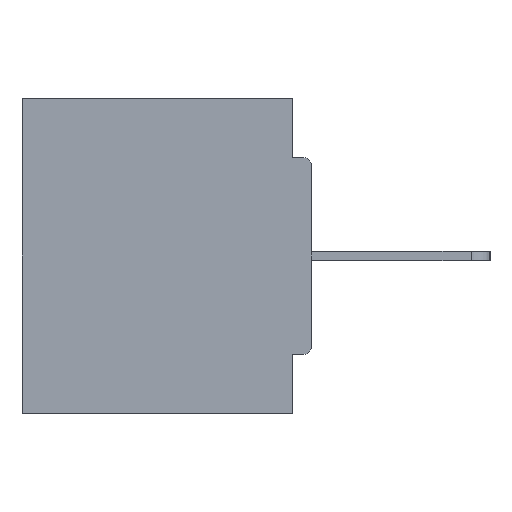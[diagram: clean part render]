
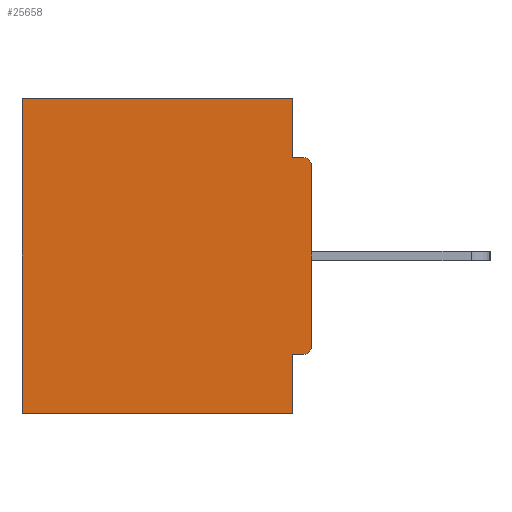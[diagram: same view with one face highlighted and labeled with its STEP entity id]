
A CAD part, left-side view. The second image highlights one B-rep face of the part: STEP entity #25658.
In plain terms, the highlighted planar face has unit normal (-1, 0, 0).
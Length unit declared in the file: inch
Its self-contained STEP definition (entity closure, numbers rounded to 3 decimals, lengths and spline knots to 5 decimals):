
#181 = ORIENTED_EDGE ( 'NONE', *, *, #11917, .T. ) ;
#790 = VECTOR ( 'NONE', #14850, 39.37008 ) ;
#1094 = VERTEX_POINT ( 'NONE', #14234 ) ;
#1147 = ORIENTED_EDGE ( 'NONE', *, *, #4278, .F. ) ;
#1227 = CARTESIAN_POINT ( 'NONE',  ( 0.298, 0., -0.0935 ) ) ;
#1301 = EDGE_CURVE ( 'NONE', #15742, #10105, #11719, .T. ) ;
#1604 = DIRECTION ( 'NONE',  ( -1., 0., 0. ) ) ;
#2246 = ORIENTED_EDGE ( 'NONE', *, *, #27350, .T. ) ;
#3933 = ORIENTED_EDGE ( 'NONE', *, *, #7257, .F. ) ;
#4278 = EDGE_CURVE ( 'NONE', #13126, #27658, #23858, .T. ) ;
#4291 = CARTESIAN_POINT ( 'NONE',  ( 0.298, 0.031, -0.5 ) ) ;
#4510 = DIRECTION ( 'NONE',  ( 0., 0., -1. ) ) ;
#5051 = CARTESIAN_POINT ( 'NONE',  ( 0.298, 0., 0. ) ) ;
#5140 = CIRCLE ( 'NONE', #22056, 0.015 ) ;
#5255 = DIRECTION ( 'NONE',  ( -1., 0., 0. ) ) ;
#5311 = CARTESIAN_POINT ( 'NONE',  ( 0.298, 0.015, -0.0935 ) ) ;
#5749 = EDGE_CURVE ( 'NONE', #11414, #7075, #10099, .T. ) ;
#6033 = FACE_OUTER_BOUND ( 'NONE', #25112, .T. ) ;
#6386 = VECTOR ( 'NONE', #26962, 39.37008 ) ;
#6812 = CARTESIAN_POINT ( 'NONE',  ( 0.298, 0.46, 0. ) ) ;
#7075 = VERTEX_POINT ( 'NONE', #27244 ) ;
#7255 = DIRECTION ( 'NONE',  ( 0., 0., -1. ) ) ;
#7257 = EDGE_CURVE ( 'NONE', #27658, #15523, #22402, .T. ) ;
#8314 = CIRCLE ( 'NONE', #8369, 0.015 ) ;
#8369 = AXIS2_PLACEMENT_3D ( 'NONE', #18197, #5255, #20356 ) ;
#8443 = CARTESIAN_POINT ( 'NONE',  ( 0.298, 0.031, -0.5 ) ) ;
#8919 = CARTESIAN_POINT ( 'NONE',  ( 0.298, 0.031, 0. ) ) ;
#9879 = VERTEX_POINT ( 'NONE', #17936 ) ;
#10099 = LINE ( 'NONE', #10907, #15210 ) ;
#10105 = VERTEX_POINT ( 'NONE', #17517 ) ;
#10907 = CARTESIAN_POINT ( 'NONE',  ( 0.298, 0.031, -0.5 ) ) ;
#10997 = ORIENTED_EDGE ( 'NONE', *, *, #22202, .T. ) ;
#11022 = VECTOR ( 'NONE', #4510, 39.37008 ) ;
#11414 = VERTEX_POINT ( 'NONE', #8919 ) ;
#11719 = LINE ( 'NONE', #27109, #12423 ) ;
#11742 = DIRECTION ( 'NONE',  ( 0., 1., 0. ) ) ;
#11917 = EDGE_CURVE ( 'NONE', #11414, #9879, #20435, .T. ) ;
#12129 = ORIENTED_EDGE ( 'NONE', *, *, #15841, .F. ) ;
#12140 = LINE ( 'NONE', #1227, #6386 ) ;
#12423 = VECTOR ( 'NONE', #23672, 39.37008 ) ;
#12634 = DIRECTION ( 'NONE',  ( 0., 1., 0. ) ) ;
#12689 = CARTESIAN_POINT ( 'NONE',  ( 0.298, 0., 0. ) ) ;
#13126 = VERTEX_POINT ( 'NONE', #16841 ) ;
#13360 = DIRECTION ( 'NONE',  ( 0., 0., -1. ) ) ;
#13546 = VECTOR ( 'NONE', #11742, 39.37008 ) ;
#14081 = VECTOR ( 'NONE', #12634, 39.37008 ) ;
#14083 = ORIENTED_EDGE ( 'NONE', *, *, #1301, .F. ) ;
#14234 = CARTESIAN_POINT ( 'NONE',  ( 0.298, 0.46, -0.5 ) ) ;
#14805 = CARTESIAN_POINT ( 'NONE',  ( 0.298, 0.015, -0.1085 ) ) ;
#14850 = DIRECTION ( 'NONE',  ( 0., 1., 0. ) ) ;
#15210 = VECTOR ( 'NONE', #23616, 39.37008 ) ;
#15523 = VERTEX_POINT ( 'NONE', #8443 ) ;
#15645 = CARTESIAN_POINT ( 'NONE',  ( 0.298, 0., -0.1085 ) ) ;
#15742 = VERTEX_POINT ( 'NONE', #15645 ) ;
#15841 = EDGE_CURVE ( 'NONE', #15523, #1094, #18590, .T. ) ;
#16500 = AXIS2_PLACEMENT_3D ( 'NONE', #5051, #20175, #7255 ) ;
#16841 = CARTESIAN_POINT ( 'NONE',  ( 0.298, 0.015, -0.4065 ) ) ;
#16942 = DIRECTION ( 'NONE',  ( 0., 0., -1. ) ) ;
#17361 = EDGE_CURVE ( 'NONE', #9879, #1094, #23072, .T. ) ;
#17476 = VECTOR ( 'NONE', #13360, 39.37008 ) ;
#17517 = CARTESIAN_POINT ( 'NONE',  ( 0.298, 0., -0.3915 ) ) ;
#17936 = CARTESIAN_POINT ( 'NONE',  ( 0.298, 0.46, 0. ) ) ;
#18197 = CARTESIAN_POINT ( 'NONE',  ( 0.298, 0.015, -0.3915 ) ) ;
#18336 = EDGE_CURVE ( 'NONE', #7075, #24596, #12140, .T. ) ;
#18590 = LINE ( 'NONE', #24448, #13546 ) ;
#19630 = CARTESIAN_POINT ( 'NONE',  ( 0.298, 0., -0.4065 ) ) ;
#20175 = DIRECTION ( 'NONE',  ( 1., 0., 0. ) ) ;
#20356 = DIRECTION ( 'NONE',  ( 0., 0., -1. ) ) ;
#20435 = LINE ( 'NONE', #12689, #14081 ) ;
#22056 = AXIS2_PLACEMENT_3D ( 'NONE', #14805, #1604, #16942 ) ;
#22157 = PLANE ( 'NONE',  #16500 ) ;
#22202 = EDGE_CURVE ( 'NONE', #15742, #24596, #5140, .T. ) ;
#22402 = LINE ( 'NONE', #4291, #11022 ) ;
#23072 = LINE ( 'NONE', #6812, #17476 ) ;
#23589 = CARTESIAN_POINT ( 'NONE',  ( 0.298, 0.031, -0.4065 ) ) ;
#23616 = DIRECTION ( 'NONE',  ( 0., 0., -1. ) ) ;
#23672 = DIRECTION ( 'NONE',  ( 0., 0., -1. ) ) ;
#23858 = LINE ( 'NONE', #19630, #790 ) ;
#24448 = CARTESIAN_POINT ( 'NONE',  ( 0.298, 0., -0.5 ) ) ;
#24596 = VERTEX_POINT ( 'NONE', #5311 ) ;
#25112 = EDGE_LOOP ( 'NONE', ( #10997, #25247, #25475, #181, #27250, #12129, #3933, #1147, #2246, #14083 ) ) ;
#25247 = ORIENTED_EDGE ( 'NONE', *, *, #18336, .F. ) ;
#25475 = ORIENTED_EDGE ( 'NONE', *, *, #5749, .F. ) ;
#25658 = ADVANCED_FACE ( 'NONE', ( #6033 ), #22157, .F. ) ;
#26962 = DIRECTION ( 'NONE',  ( 0., -1., 0. ) ) ;
#27109 = CARTESIAN_POINT ( 'NONE',  ( 0.298, 0., 0. ) ) ;
#27244 = CARTESIAN_POINT ( 'NONE',  ( 0.298, 0.031, -0.0935 ) ) ;
#27250 = ORIENTED_EDGE ( 'NONE', *, *, #17361, .T. ) ;
#27350 = EDGE_CURVE ( 'NONE', #13126, #10105, #8314, .T. ) ;
#27658 = VERTEX_POINT ( 'NONE', #23589 ) ;
